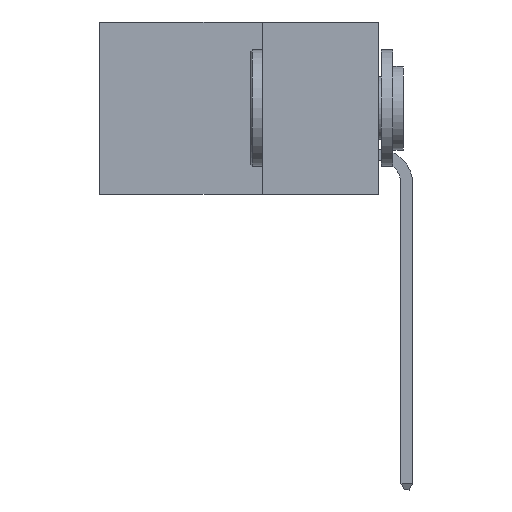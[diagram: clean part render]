
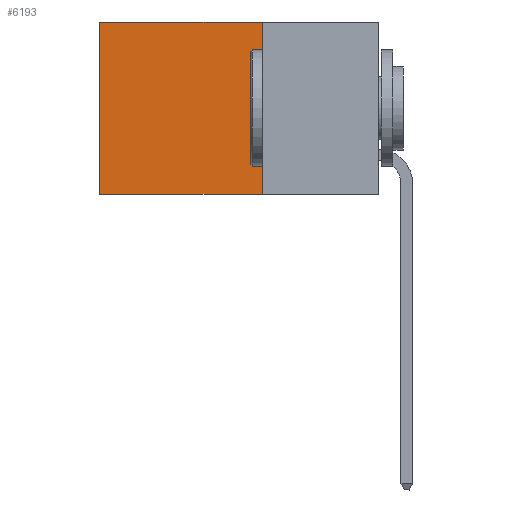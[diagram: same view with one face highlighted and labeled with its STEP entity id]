
A CAD part, left-side view. The second image highlights one B-rep face of the part: STEP entity #6193.
In plain terms, the highlighted planar face has unit normal (-1, 0, 0).
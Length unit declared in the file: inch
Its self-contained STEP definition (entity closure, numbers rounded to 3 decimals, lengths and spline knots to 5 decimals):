
#568 = CARTESIAN_POINT ( 'NONE',  ( 0.298, 0.25, 0. ) ) ;
#620 = CARTESIAN_POINT ( 'NONE',  ( 0.298, 0.25, 0. ) ) ;
#807 = VERTEX_POINT ( 'NONE', #10554 ) ;
#968 = LINE ( 'NONE', #620, #5974 ) ;
#2501 = ORIENTED_EDGE ( 'NONE', *, *, #10367, .F. ) ;
#2514 = VERTEX_POINT ( 'NONE', #568 ) ;
#2553 = CARTESIAN_POINT ( 'NONE',  ( 0.298, 0.6, 0. ) ) ;
#3156 = DIRECTION ( 'NONE',  ( 1., 0., 0. ) ) ;
#3239 = CARTESIAN_POINT ( 'NONE',  ( 0.298, 0.25, 0. ) ) ;
#3242 = ORIENTED_EDGE ( 'NONE', *, *, #4681, .T. ) ;
#3409 = VERTEX_POINT ( 'NONE', #8270 ) ;
#4681 = EDGE_CURVE ( 'NONE', #2514, #807, #968, .T. ) ;
#4757 = CARTESIAN_POINT ( 'NONE',  ( 0.298, 0.25, 0. ) ) ;
#5367 = DIRECTION ( 'NONE',  ( 0., 1., 0. ) ) ;
#5961 = EDGE_CURVE ( 'NONE', #9022, #3409, #11322, .T. ) ;
#5974 = VECTOR ( 'NONE', #5367, 39.37008 ) ;
#6193 = ADVANCED_FACE ( 'NONE', ( #10563 ), #10739, .F. ) ;
#6242 = VECTOR ( 'NONE', #10087, 39.37008 ) ;
#6370 = EDGE_CURVE ( 'NONE', #807, #3409, #10421, .T. ) ;
#6399 = VECTOR ( 'NONE', #10390, 39.37008 ) ;
#6743 = LINE ( 'NONE', #4757, #6889 ) ;
#6756 = EDGE_LOOP ( 'NONE', ( #10372, #10884, #2501, #3242 ) ) ;
#6889 = VECTOR ( 'NONE', #8437, 39.37008 ) ;
#8270 = CARTESIAN_POINT ( 'NONE',  ( 0.298, 0.6, -0.37 ) ) ;
#8437 = DIRECTION ( 'NONE',  ( 0., 0., -1. ) ) ;
#8870 = AXIS2_PLACEMENT_3D ( 'NONE', #3239, #3156, #11769 ) ;
#9022 = VERTEX_POINT ( 'NONE', #9632 ) ;
#9104 = CARTESIAN_POINT ( 'NONE',  ( 0.298, 0.25, -0.37 ) ) ;
#9632 = CARTESIAN_POINT ( 'NONE',  ( 0.298, 0.25, -0.37 ) ) ;
#10087 = DIRECTION ( 'NONE',  ( 0., 1., 0. ) ) ;
#10367 = EDGE_CURVE ( 'NONE', #2514, #9022, #6743, .T. ) ;
#10372 = ORIENTED_EDGE ( 'NONE', *, *, #6370, .T. ) ;
#10390 = DIRECTION ( 'NONE',  ( 0., 0., -1. ) ) ;
#10421 = LINE ( 'NONE', #2553, #6399 ) ;
#10554 = CARTESIAN_POINT ( 'NONE',  ( 0.298, 0.6, 0. ) ) ;
#10563 = FACE_OUTER_BOUND ( 'NONE', #6756, .T. ) ;
#10739 = PLANE ( 'NONE',  #8870 ) ;
#10884 = ORIENTED_EDGE ( 'NONE', *, *, #5961, .F. ) ;
#11322 = LINE ( 'NONE', #9104, #6242 ) ;
#11769 = DIRECTION ( 'NONE',  ( 0., 0., -1. ) ) ;
